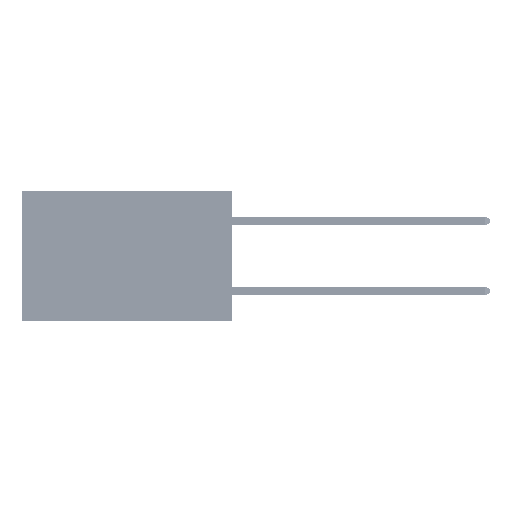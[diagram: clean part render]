
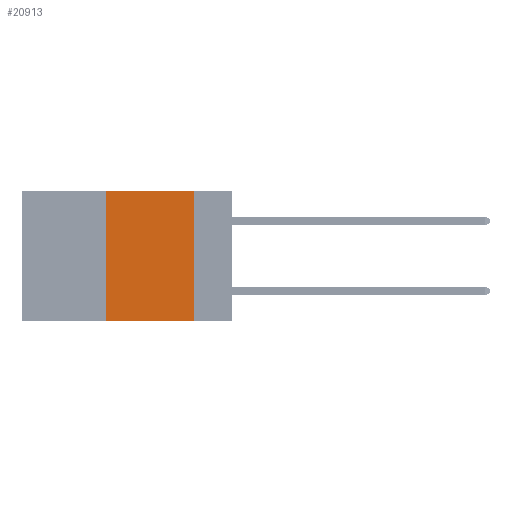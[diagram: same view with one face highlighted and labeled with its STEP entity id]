
A CAD part, left-side view. The second image highlights one B-rep face of the part: STEP entity #20913.
In plain terms, the highlighted planar face has unit normal (-1, 0, 0).
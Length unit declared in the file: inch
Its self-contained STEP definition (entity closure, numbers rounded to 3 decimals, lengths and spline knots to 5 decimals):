
#1309 = EDGE_CURVE ( 'NONE', #39208, #13692, #12460, .T. ) ;
#1775 = DIRECTION ( 'NONE',  ( 0., 0., 1. ) ) ;
#3413 = VECTOR ( 'NONE', #25093, 39.37008 ) ;
#3581 = VERTEX_POINT ( 'NONE', #28245 ) ;
#4216 = EDGE_CURVE ( 'NONE', #3581, #39208, #20432, .T. ) ;
#4704 = PLANE ( 'NONE',  #20938 ) ;
#6458 = DIRECTION ( 'NONE',  ( 0., -1., 0. ) ) ;
#12176 = CARTESIAN_POINT ( 'NONE',  ( 0., 0.6, 0. ) ) ;
#12460 = LINE ( 'NONE', #49280, #15492 ) ;
#13692 = VERTEX_POINT ( 'NONE', #41713 ) ;
#15492 = VECTOR ( 'NONE', #45210, 39.37008 ) ;
#17031 = VECTOR ( 'NONE', #1775, 39.37008 ) ;
#18256 = CARTESIAN_POINT ( 'NONE',  ( 0., 0.36, -0.37 ) ) ;
#20432 = LINE ( 'NONE', #37494, #27160 ) ;
#20913 = ADVANCED_FACE ( 'NONE', ( #35018 ), #4704, .F. ) ;
#20938 = AXIS2_PLACEMENT_3D ( 'NONE', #12176, #28187, #31434 ) ;
#23873 = EDGE_LOOP ( 'NONE', ( #48653, #46450, #33859, #44776 ) ) ;
#24694 = LINE ( 'NONE', #36875, #3413 ) ;
#25093 = DIRECTION ( 'NONE',  ( 0., -1., 0. ) ) ;
#27160 = VECTOR ( 'NONE', #6458, 39.37008 ) ;
#28187 = DIRECTION ( 'NONE',  ( 1., 0., 0. ) ) ;
#28245 = CARTESIAN_POINT ( 'NONE',  ( 0., 0.36, 0. ) ) ;
#28503 = CARTESIAN_POINT ( 'NONE',  ( 0., 0.36, 0. ) ) ;
#30204 = CARTESIAN_POINT ( 'NONE',  ( 0., 0.11, 0. ) ) ;
#31434 = DIRECTION ( 'NONE',  ( 0., 0., -1. ) ) ;
#33859 = ORIENTED_EDGE ( 'NONE', *, *, #41592, .F. ) ;
#35018 = FACE_OUTER_BOUND ( 'NONE', #23873, .T. ) ;
#36875 = CARTESIAN_POINT ( 'NONE',  ( 0., 0.6, -0.37 ) ) ;
#37222 = VERTEX_POINT ( 'NONE', #18256 ) ;
#37494 = CARTESIAN_POINT ( 'NONE',  ( 0., 0.6, 0. ) ) ;
#37807 = LINE ( 'NONE', #28503, #17031 ) ;
#39208 = VERTEX_POINT ( 'NONE', #30204 ) ;
#39568 = EDGE_CURVE ( 'NONE', #37222, #13692, #24694, .T. ) ;
#41592 = EDGE_CURVE ( 'NONE', #37222, #3581, #37807, .T. ) ;
#41713 = CARTESIAN_POINT ( 'NONE',  ( 0., 0.11, -0.37 ) ) ;
#44776 = ORIENTED_EDGE ( 'NONE', *, *, #39568, .T. ) ;
#45210 = DIRECTION ( 'NONE',  ( 0., 0., -1. ) ) ;
#46450 = ORIENTED_EDGE ( 'NONE', *, *, #4216, .F. ) ;
#48653 = ORIENTED_EDGE ( 'NONE', *, *, #1309, .F. ) ;
#49280 = CARTESIAN_POINT ( 'NONE',  ( 0., 0.11, 0. ) ) ;
